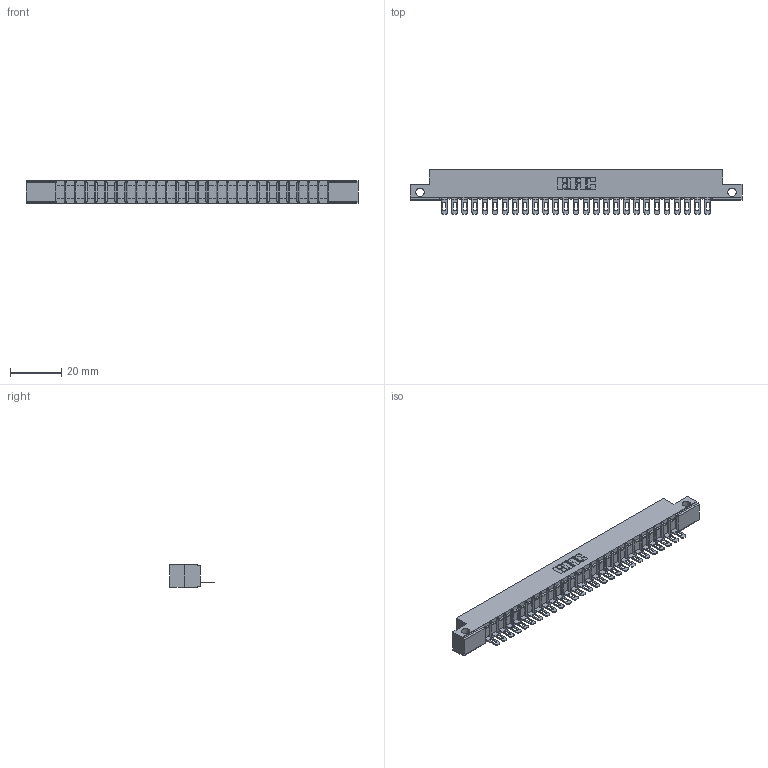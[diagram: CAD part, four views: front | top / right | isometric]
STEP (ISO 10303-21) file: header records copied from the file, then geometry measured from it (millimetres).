
FILE_DESCRIPTION (( 'STEP AP203' ), '1' );
FILE_NAME ('307-027-401-112.STEP', '2020-09-28T05:16:01', ( '' ), ( '' ), 'SwSTEP 2.0', 'SolidWorks 2020', '' );
FILE_SCHEMA (( 'CONFIG_CONTROL_DESIGN' ));
Length unit declared in the file: inch
Products named in the file (3): 307-027-401-112; 307 Part_.128 Dia Side Mounting Holes; 307-290-002_501
Assembly tree (28 placements, depth 2):
  307-027-401-112
    307 Part_.128 Dia Side Mounting Holes
    307-290-002_501  x27
Bounding box: 130 x 17.42 x 8.71 mm (x, y, z)
Volume: 8532.4 mm3; surface area: 15841.2 mm2
Topology: 28 solids, 28 shells, 2198 faces, 6749 edges, 4422 vertices
Faces by surface type: plane 1258, cylinder 884, sphere 56
Entity records: 25792 total; most frequent: CARTESIAN_POINT 4348, ORIENTED_EDGE 4338, DIRECTION 4235, EDGE_CURVE 2169, VECTOR 1649, LINE 1649, VERTEX_POINT 1406, AXIS2_PLACEMENT_3D 1293
